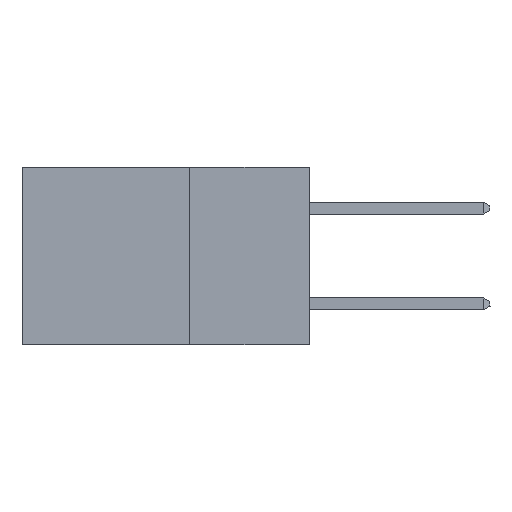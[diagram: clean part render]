
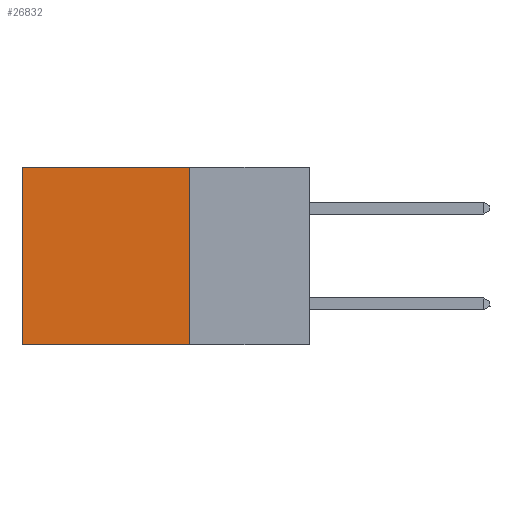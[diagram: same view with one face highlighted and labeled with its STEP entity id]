
A CAD part, left-side view. The second image highlights one B-rep face of the part: STEP entity #26832.
In plain terms, the highlighted planar face has unit normal (-1, 0, 0).
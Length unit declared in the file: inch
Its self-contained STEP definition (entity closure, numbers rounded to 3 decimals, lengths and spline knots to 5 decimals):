
#1968 = DIRECTION ( 'NONE',  ( 0., 1., 0. ) ) ;
#2771 = CARTESIAN_POINT ( 'NONE',  ( 0.2875, 0.6, -0.37 ) ) ;
#3212 = CARTESIAN_POINT ( 'NONE',  ( 0.2875, 0.25, 0. ) ) ;
#3243 = VERTEX_POINT ( 'NONE', #24573 ) ;
#3768 = CARTESIAN_POINT ( 'NONE',  ( 0.2875, 0.25, -0.37 ) ) ;
#3969 = ORIENTED_EDGE ( 'NONE', *, *, #18315, .T. ) ;
#4672 = VECTOR ( 'NONE', #4967, 39.37008 ) ;
#4967 = DIRECTION ( 'NONE',  ( 0., 0., -1. ) ) ;
#5408 = DIRECTION ( 'NONE',  ( 0., 0., -1. ) ) ;
#8379 = VECTOR ( 'NONE', #5408, 39.37008 ) ;
#8516 = DIRECTION ( 'NONE',  ( 0., 1., 0. ) ) ;
#9824 = DIRECTION ( 'NONE',  ( 0., 0., -1. ) ) ;
#10037 = PLANE ( 'NONE',  #17682 ) ;
#12257 = ORIENTED_EDGE ( 'NONE', *, *, #28175, .T. ) ;
#15177 = CARTESIAN_POINT ( 'NONE',  ( 0.2875, 0.25, 0. ) ) ;
#15434 = EDGE_LOOP ( 'NONE', ( #3969, #27672, #29088, #12257 ) ) ;
#15852 = VECTOR ( 'NONE', #1968, 39.37008 ) ;
#15886 = LINE ( 'NONE', #3768, #31844 ) ;
#16000 = LINE ( 'NONE', #3212, #8379 ) ;
#16657 = LINE ( 'NONE', #17197, #15852 ) ;
#17197 = CARTESIAN_POINT ( 'NONE',  ( 0.2875, 0.25, 0. ) ) ;
#17682 = AXIS2_PLACEMENT_3D ( 'NONE', #15177, #25040, #9824 ) ;
#18315 = EDGE_CURVE ( 'NONE', #3243, #28989, #28205, .T. ) ;
#19614 = VERTEX_POINT ( 'NONE', #23894 ) ;
#20072 = EDGE_CURVE ( 'NONE', #27172, #19614, #16000, .T. ) ;
#21421 = EDGE_CURVE ( 'NONE', #19614, #28989, #15886, .T. ) ;
#22004 = FACE_OUTER_BOUND ( 'NONE', #15434, .T. ) ;
#23894 = CARTESIAN_POINT ( 'NONE',  ( 0.2875, 0.25, -0.37 ) ) ;
#24573 = CARTESIAN_POINT ( 'NONE',  ( 0.2875, 0.6, 0. ) ) ;
#25040 = DIRECTION ( 'NONE',  ( 1., 0., 0. ) ) ;
#26832 = ADVANCED_FACE ( 'NONE', ( #22004 ), #10037, .F. ) ;
#27172 = VERTEX_POINT ( 'NONE', #28120 ) ;
#27672 = ORIENTED_EDGE ( 'NONE', *, *, #21421, .F. ) ;
#28120 = CARTESIAN_POINT ( 'NONE',  ( 0.2875, 0.25, 0. ) ) ;
#28175 = EDGE_CURVE ( 'NONE', #27172, #3243, #16657, .T. ) ;
#28205 = LINE ( 'NONE', #32924, #4672 ) ;
#28989 = VERTEX_POINT ( 'NONE', #2771 ) ;
#29088 = ORIENTED_EDGE ( 'NONE', *, *, #20072, .F. ) ;
#31844 = VECTOR ( 'NONE', #8516, 39.37008 ) ;
#32924 = CARTESIAN_POINT ( 'NONE',  ( 0.2875, 0.6, 0. ) ) ;
